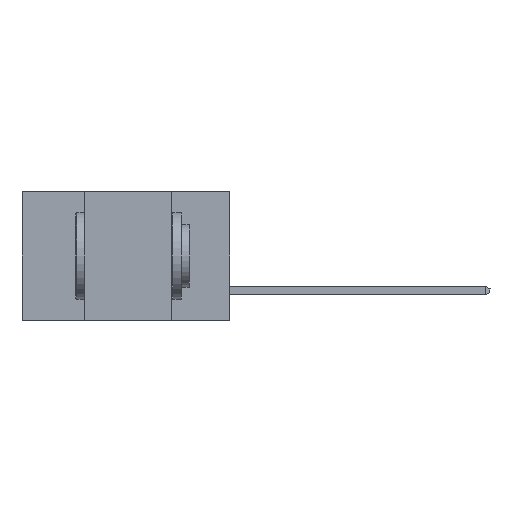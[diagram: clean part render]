
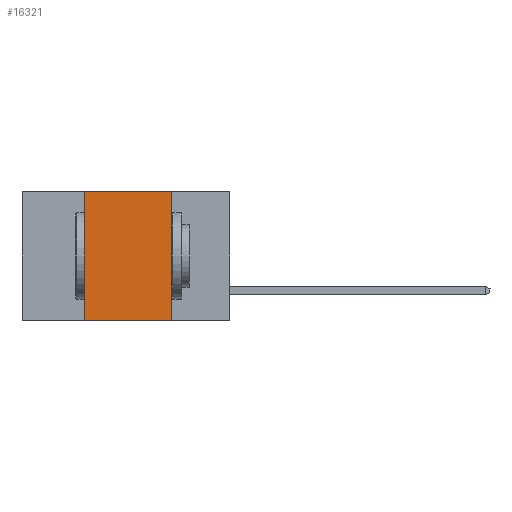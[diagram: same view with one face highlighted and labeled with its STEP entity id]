
A CAD part, left-side view. The second image highlights one B-rep face of the part: STEP entity #16321.
In plain terms, the highlighted planar face has unit normal (-1, 0, 0).
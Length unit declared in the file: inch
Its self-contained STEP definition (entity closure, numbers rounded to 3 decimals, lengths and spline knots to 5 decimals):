
#739 = DIRECTION ( 'NONE',  ( 0., 0., -1. ) ) ;
#2595 = VECTOR ( 'NONE', #3060, 39.37008 ) ;
#2761 = FACE_OUTER_BOUND ( 'NONE', #17910, .T. ) ;
#3060 = DIRECTION ( 'NONE',  ( 0., 0., 1. ) ) ;
#4739 = CARTESIAN_POINT ( 'NONE',  ( 0., 0.17, -0.37 ) ) ;
#5912 = LINE ( 'NONE', #9598, #18622 ) ;
#5963 = CARTESIAN_POINT ( 'NONE',  ( 0., 0.42, 0. ) ) ;
#6564 = DIRECTION ( 'NONE',  ( 1., 0., 0. ) ) ;
#7508 = LINE ( 'NONE', #11171, #24678 ) ;
#7819 = CARTESIAN_POINT ( 'NONE',  ( 0., 0.6, 0. ) ) ;
#7872 = CARTESIAN_POINT ( 'NONE',  ( 0., 0.17, 0. ) ) ;
#7968 = EDGE_CURVE ( 'NONE', #14295, #20913, #16604, .T. ) ;
#8085 = ORIENTED_EDGE ( 'NONE', *, *, #10165, .F. ) ;
#8111 = VERTEX_POINT ( 'NONE', #7872 ) ;
#9597 = DIRECTION ( 'NONE',  ( 0., -1., 0. ) ) ;
#9598 = CARTESIAN_POINT ( 'NONE',  ( 0., 0.6, -0.37 ) ) ;
#9975 = DIRECTION ( 'NONE',  ( 0., -1., 0. ) ) ;
#10165 = EDGE_CURVE ( 'NONE', #8111, #18555, #7508, .T. ) ;
#11171 = CARTESIAN_POINT ( 'NONE',  ( 0., 0.17, -0.37 ) ) ;
#12609 = ORIENTED_EDGE ( 'NONE', *, *, #7968, .F. ) ;
#12962 = ORIENTED_EDGE ( 'NONE', *, *, #17875, .F. ) ;
#12981 = ORIENTED_EDGE ( 'NONE', *, *, #24836, .T. ) ;
#14295 = VERTEX_POINT ( 'NONE', #22855 ) ;
#14834 = CARTESIAN_POINT ( 'NONE',  ( 0., 0.42, -0.37 ) ) ;
#16321 = ADVANCED_FACE ( 'NONE', ( #2761 ), #18346, .F. ) ;
#16445 = CARTESIAN_POINT ( 'NONE',  ( 0., 0.6, 0. ) ) ;
#16604 = LINE ( 'NONE', #14834, #2595 ) ;
#17689 = LINE ( 'NONE', #7819, #19674 ) ;
#17875 = EDGE_CURVE ( 'NONE', #20913, #8111, #17689, .T. ) ;
#17910 = EDGE_LOOP ( 'NONE', ( #8085, #12962, #12609, #12981 ) ) ;
#18346 = PLANE ( 'NONE',  #22469 ) ;
#18555 = VERTEX_POINT ( 'NONE', #4739 ) ;
#18622 = VECTOR ( 'NONE', #9975, 39.37008 ) ;
#19398 = DIRECTION ( 'NONE',  ( 0., 0., -1. ) ) ;
#19674 = VECTOR ( 'NONE', #9597, 39.37008 ) ;
#20913 = VERTEX_POINT ( 'NONE', #5963 ) ;
#22469 = AXIS2_PLACEMENT_3D ( 'NONE', #16445, #6564, #739 ) ;
#22855 = CARTESIAN_POINT ( 'NONE',  ( 0., 0.42, -0.37 ) ) ;
#24678 = VECTOR ( 'NONE', #19398, 39.37008 ) ;
#24836 = EDGE_CURVE ( 'NONE', #14295, #18555, #5912, .T. ) ;
